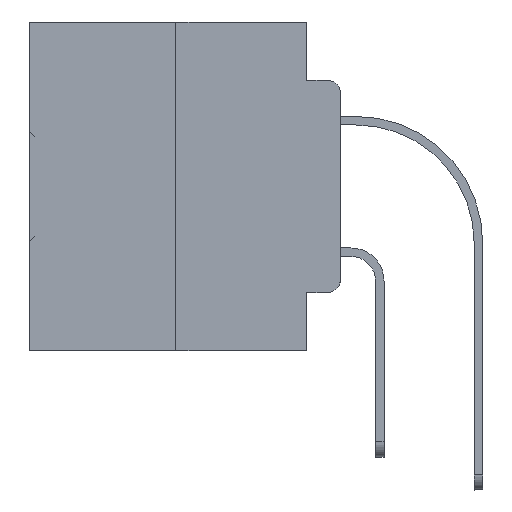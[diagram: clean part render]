
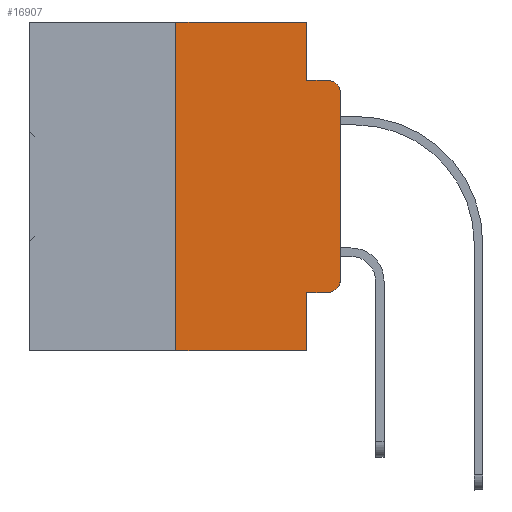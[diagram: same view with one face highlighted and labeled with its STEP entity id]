
A CAD part, left-side view. The second image highlights one B-rep face of the part: STEP entity #16907.
In plain terms, the highlighted planar face has unit normal (-1, 0, 0).
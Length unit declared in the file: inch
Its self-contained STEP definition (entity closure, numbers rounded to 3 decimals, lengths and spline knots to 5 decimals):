
#79 = CARTESIAN_POINT ( 'NONE',  ( 0., 0.051, 0. ) ) ;
#838 = DIRECTION ( 'NONE',  ( 0., -1., 0. ) ) ;
#1956 = CARTESIAN_POINT ( 'NONE',  ( 0., 0., -0.3915 ) ) ;
#1983 = VECTOR ( 'NONE', #24212, 39.37008 ) ;
#2318 = VECTOR ( 'NONE', #9554, 39.37008 ) ;
#2420 = EDGE_CURVE ( 'NONE', #10175, #32442, #3754, .T. ) ;
#2530 = DIRECTION ( 'NONE',  ( 1., 0., 0. ) ) ;
#2721 = FACE_OUTER_BOUND ( 'NONE', #26845, .T. ) ;
#3070 = EDGE_CURVE ( 'NONE', #5464, #35223, #12190, .T. ) ;
#3282 = DIRECTION ( 'NONE',  ( 0., -1., 0. ) ) ;
#3554 = CARTESIAN_POINT ( 'NONE',  ( 0., 0.02, -0.3915 ) ) ;
#3731 = ORIENTED_EDGE ( 'NONE', *, *, #24683, .F. ) ;
#3754 = LINE ( 'NONE', #9033, #17967 ) ;
#3757 = DIRECTION ( 'NONE',  ( 0., 0., -1. ) ) ;
#4053 = DIRECTION ( 'NONE',  ( 0., -1., 0. ) ) ;
#4592 = LINE ( 'NONE', #24322, #2318 ) ;
#5451 = PLANE ( 'NONE',  #15590 ) ;
#5464 = VERTEX_POINT ( 'NONE', #16306 ) ;
#5471 = VECTOR ( 'NONE', #32807, 39.37008 ) ;
#5838 = DIRECTION ( 'NONE',  ( 0., 0., -1. ) ) ;
#6333 = LINE ( 'NONE', #18179, #24984 ) ;
#6688 = DIRECTION ( 'NONE',  ( -1., 0., 0. ) ) ;
#7029 = LINE ( 'NONE', #30555, #19955 ) ;
#7799 = EDGE_CURVE ( 'NONE', #5464, #36179, #4592, .T. ) ;
#8426 = ORIENTED_EDGE ( 'NONE', *, *, #3070, .F. ) ;
#8750 = ORIENTED_EDGE ( 'NONE', *, *, #37580, .T. ) ;
#8871 = CARTESIAN_POINT ( 'NONE',  ( 0., 0.25, 0. ) ) ;
#9033 = CARTESIAN_POINT ( 'NONE',  ( 0., 0.051, -0.0885 ) ) ;
#9554 = DIRECTION ( 'NONE',  ( 0., -1., 0. ) ) ;
#10175 = VERTEX_POINT ( 'NONE', #23754 ) ;
#10749 = DIRECTION ( 'NONE',  ( 0., 0., -1. ) ) ;
#12190 = LINE ( 'NONE', #29888, #5471 ) ;
#12221 = VERTEX_POINT ( 'NONE', #79 ) ;
#13850 = CARTESIAN_POINT ( 'NONE',  ( 0., 0.02, -0.1085 ) ) ;
#14594 = EDGE_CURVE ( 'NONE', #33887, #12221, #30712, .T. ) ;
#15446 = CARTESIAN_POINT ( 'NONE',  ( 0., 0.25, 0. ) ) ;
#15590 = AXIS2_PLACEMENT_3D ( 'NONE', #23158, #2530, #5838 ) ;
#16119 = VECTOR ( 'NONE', #4053, 39.37008 ) ;
#16168 = VERTEX_POINT ( 'NONE', #36676 ) ;
#16306 = CARTESIAN_POINT ( 'NONE',  ( 0., 0.051, -0.4115 ) ) ;
#16907 = ADVANCED_FACE ( 'NONE', ( #2721 ), #5451, .F. ) ;
#17339 = CIRCLE ( 'NONE', #18576, 0.02 ) ;
#17967 = VECTOR ( 'NONE', #838, 39.37008 ) ;
#18179 = CARTESIAN_POINT ( 'NONE',  ( 0., 0., 0. ) ) ;
#18187 = ORIENTED_EDGE ( 'NONE', *, *, #19251, .F. ) ;
#18576 = AXIS2_PLACEMENT_3D ( 'NONE', #13850, #20058, #10749 ) ;
#18848 = CARTESIAN_POINT ( 'NONE',  ( 0., 0.02, -0.4115 ) ) ;
#18860 = DIRECTION ( 'NONE',  ( 0., 0., -1. ) ) ;
#19016 = VERTEX_POINT ( 'NONE', #19549 ) ;
#19234 = EDGE_CURVE ( 'NONE', #32735, #16168, #6333, .T. ) ;
#19251 = EDGE_CURVE ( 'NONE', #19016, #33887, #21286, .T. ) ;
#19368 = AXIS2_PLACEMENT_3D ( 'NONE', #3554, #6688, #3757 ) ;
#19549 = CARTESIAN_POINT ( 'NONE',  ( 0., 0.25, -0.5 ) ) ;
#19955 = VECTOR ( 'NONE', #18860, 39.37008 ) ;
#20058 = DIRECTION ( 'NONE',  ( -1., 0., 0. ) ) ;
#20201 = ORIENTED_EDGE ( 'NONE', *, *, #19234, .T. ) ;
#21286 = LINE ( 'NONE', #15446, #1983 ) ;
#21291 = VECTOR ( 'NONE', #3282, 39.37008 ) ;
#22437 = CARTESIAN_POINT ( 'NONE',  ( 0., 0.051, -0.5 ) ) ;
#23158 = CARTESIAN_POINT ( 'NONE',  ( 0., 0.473, 0. ) ) ;
#23754 = CARTESIAN_POINT ( 'NONE',  ( 0., 0.051, -0.0885 ) ) ;
#23913 = ORIENTED_EDGE ( 'NONE', *, *, #14594, .F. ) ;
#24212 = DIRECTION ( 'NONE',  ( 0., 0., 1. ) ) ;
#24322 = CARTESIAN_POINT ( 'NONE',  ( 0., 0.051, -0.4115 ) ) ;
#24683 = EDGE_CURVE ( 'NONE', #12221, #10175, #7029, .T. ) ;
#24984 = VECTOR ( 'NONE', #35723, 39.37008 ) ;
#26845 = EDGE_LOOP ( 'NONE', ( #20201, #29913, #33736, #3731, #23913, #18187, #8750, #8426, #30769, #33111 ) ) ;
#27233 = EDGE_CURVE ( 'NONE', #36179, #32735, #28166, .T. ) ;
#27499 = CARTESIAN_POINT ( 'NONE',  ( 0., 0.02, -0.0885 ) ) ;
#28166 = CIRCLE ( 'NONE', #19368, 0.02 ) ;
#29888 = CARTESIAN_POINT ( 'NONE',  ( 0., 0.051, 0. ) ) ;
#29913 = ORIENTED_EDGE ( 'NONE', *, *, #35852, .T. ) ;
#30124 = CARTESIAN_POINT ( 'NONE',  ( 0., 0.473, -0.5 ) ) ;
#30555 = CARTESIAN_POINT ( 'NONE',  ( 0., 0.051, 0. ) ) ;
#30712 = LINE ( 'NONE', #34043, #16119 ) ;
#30769 = ORIENTED_EDGE ( 'NONE', *, *, #7799, .T. ) ;
#31513 = LINE ( 'NONE', #30124, #21291 ) ;
#32442 = VERTEX_POINT ( 'NONE', #27499 ) ;
#32735 = VERTEX_POINT ( 'NONE', #1956 ) ;
#32807 = DIRECTION ( 'NONE',  ( 0., 0., -1. ) ) ;
#33111 = ORIENTED_EDGE ( 'NONE', *, *, #27233, .T. ) ;
#33736 = ORIENTED_EDGE ( 'NONE', *, *, #2420, .F. ) ;
#33887 = VERTEX_POINT ( 'NONE', #8871 ) ;
#34043 = CARTESIAN_POINT ( 'NONE',  ( 0., 0.473, 0. ) ) ;
#35223 = VERTEX_POINT ( 'NONE', #22437 ) ;
#35723 = DIRECTION ( 'NONE',  ( 0., 0., 1. ) ) ;
#35852 = EDGE_CURVE ( 'NONE', #16168, #32442, #17339, .T. ) ;
#36179 = VERTEX_POINT ( 'NONE', #18848 ) ;
#36676 = CARTESIAN_POINT ( 'NONE',  ( 0., 0., -0.1085 ) ) ;
#37580 = EDGE_CURVE ( 'NONE', #19016, #35223, #31513, .T. ) ;
